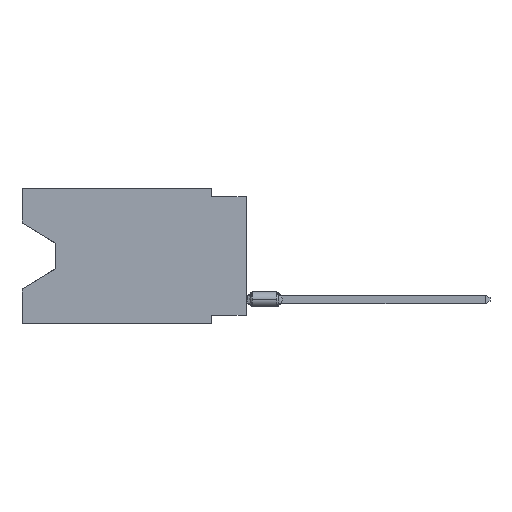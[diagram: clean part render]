
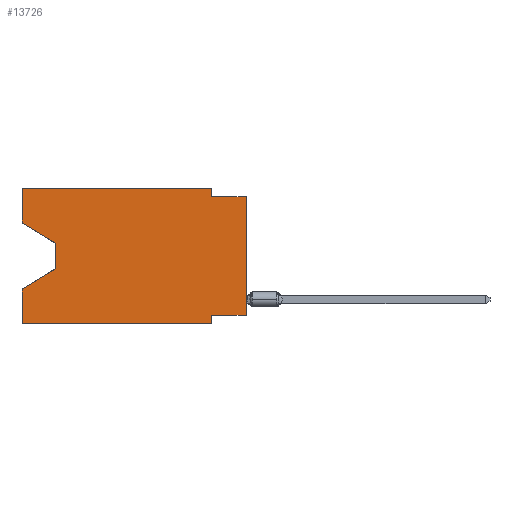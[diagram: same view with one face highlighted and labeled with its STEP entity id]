
A CAD part, left-side view. The second image highlights one B-rep face of the part: STEP entity #13726.
In plain terms, the highlighted planar face has unit normal (-1, 0, 0).
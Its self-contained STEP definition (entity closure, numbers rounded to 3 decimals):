
#258 = ORIENTED_EDGE ( 'NONE', *, *, #16746, .F. ) ;
#419 = EDGE_CURVE ( 'NONE', #23504, #15532, #6134, .T. ) ;
#446 = CARTESIAN_POINT ( 'NONE',  ( 0., 13.97, -4.013 ) ) ;
#1050 = DIRECTION ( 'NONE',  ( 0., 0., -1. ) ) ;
#1161 = ORIENTED_EDGE ( 'NONE', *, *, #20347, .F. ) ;
#1305 = CARTESIAN_POINT ( 'NONE',  ( 0., 16.383, -2.546 ) ) ;
#1376 = EDGE_LOOP ( 'NONE', ( #7511, #6923, #2861, #22818, #17700, #11758, #1161, #5635, #258, #18103, #22439, #5272 ) ) ;
#1413 = VECTOR ( 'NONE', #6223, 1000. ) ;
#1663 = CARTESIAN_POINT ( 'NONE',  ( 0., 16.383, -7.36 ) ) ;
#1966 = CARTESIAN_POINT ( 'NONE',  ( 0., 2.54, -9.906 ) ) ;
#2007 = CARTESIAN_POINT ( 'NONE',  ( 0., 0., -0.635 ) ) ;
#2160 = LINE ( 'NONE', #10756, #16907 ) ;
#2201 = DIRECTION ( 'NONE',  ( 0., 0.855, -0.519 ) ) ;
#2566 = VECTOR ( 'NONE', #5890, 1000. ) ;
#2780 = DIRECTION ( 'NONE',  ( 0., 0., 1. ) ) ;
#2861 = ORIENTED_EDGE ( 'NONE', *, *, #5189, .T. ) ;
#3151 = VECTOR ( 'NONE', #18499, 1000. ) ;
#3899 = VERTEX_POINT ( 'NONE', #19664 ) ;
#4407 = DIRECTION ( 'NONE',  ( 0., -1., 0. ) ) ;
#4431 = DIRECTION ( 'NONE',  ( 0., -1., 0. ) ) ;
#4774 = LINE ( 'NONE', #13375, #17625 ) ;
#5189 = EDGE_CURVE ( 'NONE', #5600, #22493, #21364, .T. ) ;
#5272 = ORIENTED_EDGE ( 'NONE', *, *, #12078, .F. ) ;
#5537 = VECTOR ( 'NONE', #4407, 1000. ) ;
#5600 = VERTEX_POINT ( 'NONE', #8326 ) ;
#5635 = ORIENTED_EDGE ( 'NONE', *, *, #26504, .T. ) ;
#5849 = CARTESIAN_POINT ( 'NONE',  ( 0., 16.383, -9.906 ) ) ;
#5890 = DIRECTION ( 'NONE',  ( 0., 0., 1. ) ) ;
#6134 = LINE ( 'NONE', #18656, #3151 ) ;
#6223 = DIRECTION ( 'NONE',  ( 0., 0., 1. ) ) ;
#6247 = CARTESIAN_POINT ( 'NONE',  ( 0., 16.383, 0. ) ) ;
#6253 = CARTESIAN_POINT ( 'NONE',  ( 0., 0., -0.635 ) ) ;
#6736 = DIRECTION ( 'NONE',  ( 0., 0., -1. ) ) ;
#6923 = ORIENTED_EDGE ( 'NONE', *, *, #14497, .T. ) ;
#7302 = CARTESIAN_POINT ( 'NONE',  ( 0., 13.97, -4.013 ) ) ;
#7411 = CARTESIAN_POINT ( 'NONE',  ( 0., 0., -9.271 ) ) ;
#7511 = ORIENTED_EDGE ( 'NONE', *, *, #23162, .T. ) ;
#7720 = EDGE_CURVE ( 'NONE', #9389, #8277, #21262, .T. ) ;
#7955 = VERTEX_POINT ( 'NONE', #5849 ) ;
#8277 = VERTEX_POINT ( 'NONE', #9905 ) ;
#8326 = CARTESIAN_POINT ( 'NONE',  ( 0., 13.97, -5.893 ) ) ;
#8357 = LINE ( 'NONE', #6247, #22313 ) ;
#8843 = CARTESIAN_POINT ( 'NONE',  ( 0., 13.97, -5.893 ) ) ;
#9331 = AXIS2_PLACEMENT_3D ( 'NONE', #13610, #22057, #1050 ) ;
#9389 = VERTEX_POINT ( 'NONE', #13362 ) ;
#9711 = LINE ( 'NONE', #7302, #12957 ) ;
#9905 = CARTESIAN_POINT ( 'NONE',  ( 0., 2.54, -9.906 ) ) ;
#10058 = DIRECTION ( 'NONE',  ( 0., -0.855, -0.519 ) ) ;
#10460 = DIRECTION ( 'NONE',  ( 0., -1., 0. ) ) ;
#10756 = CARTESIAN_POINT ( 'NONE',  ( 0., 0., -9.271 ) ) ;
#11082 = LINE ( 'NONE', #27442, #2566 ) ;
#11595 = CARTESIAN_POINT ( 'NONE',  ( 0., 2.54, 0. ) ) ;
#11758 = ORIENTED_EDGE ( 'NONE', *, *, #7720, .F. ) ;
#12078 = EDGE_CURVE ( 'NONE', #27082, #3899, #4774, .T. ) ;
#12447 = VECTOR ( 'NONE', #4431, 1000. ) ;
#12712 = CARTESIAN_POINT ( 'NONE',  ( 0., 2.54, -0.635 ) ) ;
#12830 = VERTEX_POINT ( 'NONE', #446 ) ;
#12957 = VECTOR ( 'NONE', #14061, 1000. ) ;
#13142 = LINE ( 'NONE', #2007, #5537 ) ;
#13357 = EDGE_CURVE ( 'NONE', #7955, #22493, #11082, .T. ) ;
#13362 = CARTESIAN_POINT ( 'NONE',  ( 0., 2.54, -9.271 ) ) ;
#13375 = CARTESIAN_POINT ( 'NONE',  ( 0., 16.383, 0. ) ) ;
#13610 = CARTESIAN_POINT ( 'NONE',  ( 0., 16.383, 0. ) ) ;
#13726 = ADVANCED_FACE ( 'NONE', ( #13893 ), #22470, .F. ) ;
#13789 = VERTEX_POINT ( 'NONE', #7411 ) ;
#13893 = FACE_OUTER_BOUND ( 'NONE', #1376, .T. ) ;
#14061 = DIRECTION ( 'NONE',  ( 0., 0., -1. ) ) ;
#14063 = EDGE_CURVE ( 'NONE', #7955, #8277, #15162, .T. ) ;
#14497 = EDGE_CURVE ( 'NONE', #12830, #5600, #9711, .T. ) ;
#15162 = LINE ( 'NONE', #23736, #12447 ) ;
#15345 = CARTESIAN_POINT ( 'NONE',  ( 0., 16.383, -2.546 ) ) ;
#15532 = VERTEX_POINT ( 'NONE', #12712 ) ;
#15563 = EDGE_CURVE ( 'NONE', #3899, #23504, #8357, .T. ) ;
#16746 = EDGE_CURVE ( 'NONE', #15532, #19001, #13142, .T. ) ;
#16907 = VECTOR ( 'NONE', #27247, 1000. ) ;
#17625 = VECTOR ( 'NONE', #2780, 1000. ) ;
#17700 = ORIENTED_EDGE ( 'NONE', *, *, #14063, .T. ) ;
#18103 = ORIENTED_EDGE ( 'NONE', *, *, #419, .F. ) ;
#18499 = DIRECTION ( 'NONE',  ( 0., 0., -1. ) ) ;
#18656 = CARTESIAN_POINT ( 'NONE',  ( 0., 2.54, 0. ) ) ;
#19001 = VERTEX_POINT ( 'NONE', #6253 ) ;
#19664 = CARTESIAN_POINT ( 'NONE',  ( 0., 16.383, 0. ) ) ;
#20027 = VECTOR ( 'NONE', #2201, 1000. ) ;
#20347 = EDGE_CURVE ( 'NONE', #13789, #9389, #2160, .T. ) ;
#20896 = LINE ( 'NONE', #1305, #25900 ) ;
#21262 = LINE ( 'NONE', #1966, #26154 ) ;
#21271 = LINE ( 'NONE', #25509, #1413 ) ;
#21364 = LINE ( 'NONE', #8843, #20027 ) ;
#22057 = DIRECTION ( 'NONE',  ( 1., 0., 0. ) ) ;
#22313 = VECTOR ( 'NONE', #10460, 1000. ) ;
#22439 = ORIENTED_EDGE ( 'NONE', *, *, #15563, .F. ) ;
#22470 = PLANE ( 'NONE',  #9331 ) ;
#22493 = VERTEX_POINT ( 'NONE', #1663 ) ;
#22818 = ORIENTED_EDGE ( 'NONE', *, *, #13357, .F. ) ;
#23162 = EDGE_CURVE ( 'NONE', #27082, #12830, #20896, .T. ) ;
#23504 = VERTEX_POINT ( 'NONE', #11595 ) ;
#23736 = CARTESIAN_POINT ( 'NONE',  ( 0., 16.383, -9.906 ) ) ;
#25509 = CARTESIAN_POINT ( 'NONE',  ( 0., 0., 0. ) ) ;
#25900 = VECTOR ( 'NONE', #10058, 1000. ) ;
#26154 = VECTOR ( 'NONE', #6736, 1000. ) ;
#26504 = EDGE_CURVE ( 'NONE', #13789, #19001, #21271, .T. ) ;
#27082 = VERTEX_POINT ( 'NONE', #15345 ) ;
#27247 = DIRECTION ( 'NONE',  ( 0., 1., 0. ) ) ;
#27442 = CARTESIAN_POINT ( 'NONE',  ( 0., 16.383, 0. ) ) ;
